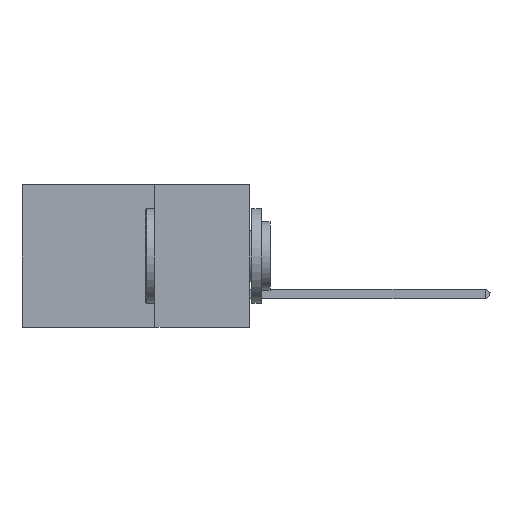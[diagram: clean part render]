
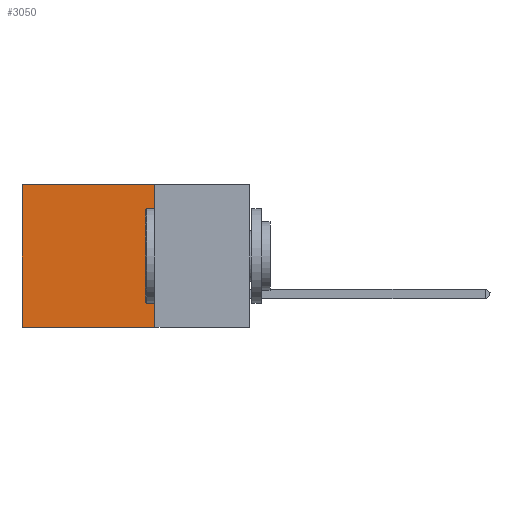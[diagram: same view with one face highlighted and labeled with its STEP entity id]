
A CAD part, left-side view. The second image highlights one B-rep face of the part: STEP entity #3050.
In plain terms, the highlighted planar face has unit normal (-1, 0, 0).
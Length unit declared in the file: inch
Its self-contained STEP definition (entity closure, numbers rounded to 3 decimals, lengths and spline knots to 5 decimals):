
#514 = DIRECTION ( 'NONE',  ( 0., 0., -1. ) ) ;
#1118 = VECTOR ( 'NONE', #9694, 39.37008 ) ;
#1240 = CARTESIAN_POINT ( 'NONE',  ( 0.2875, 0.6, -0.375 ) ) ;
#1529 = ORIENTED_EDGE ( 'NONE', *, *, #11864, .F. ) ;
#1960 = VERTEX_POINT ( 'NONE', #14443 ) ;
#3050 = ADVANCED_FACE ( 'NONE', ( #8860 ), #10366, .F. ) ;
#4208 = EDGE_LOOP ( 'NONE', ( #14770, #6728, #1529, #16789 ) ) ;
#4593 = CARTESIAN_POINT ( 'NONE',  ( 0.2875, 0.25, -0.375 ) ) ;
#5325 = EDGE_CURVE ( 'NONE', #17146, #1960, #9443, .T. ) ;
#5457 = CARTESIAN_POINT ( 'NONE',  ( 0.2875, 0.25, 0. ) ) ;
#6728 = ORIENTED_EDGE ( 'NONE', *, *, #14338, .F. ) ;
#6798 = CARTESIAN_POINT ( 'NONE',  ( 0.2875, 0.25, 0. ) ) ;
#7000 = AXIS2_PLACEMENT_3D ( 'NONE', #9120, #14892, #514 ) ;
#7699 = VERTEX_POINT ( 'NONE', #15170 ) ;
#7794 = CARTESIAN_POINT ( 'NONE',  ( 0.2875, 0.25, -0.375 ) ) ;
#7852 = VECTOR ( 'NONE', #16103, 39.37008 ) ;
#8070 = VERTEX_POINT ( 'NONE', #7794 ) ;
#8860 = FACE_OUTER_BOUND ( 'NONE', #4208, .T. ) ;
#9120 = CARTESIAN_POINT ( 'NONE',  ( 0.2875, 0.25, -0.375 ) ) ;
#9443 = LINE ( 'NONE', #6798, #1118 ) ;
#9694 = DIRECTION ( 'NONE',  ( 0., 1., 0. ) ) ;
#9783 = DIRECTION ( 'NONE',  ( 0., 0., -1. ) ) ;
#9868 = VECTOR ( 'NONE', #9783, 39.37008 ) ;
#10366 = PLANE ( 'NONE',  #7000 ) ;
#11656 = VECTOR ( 'NONE', #17622, 39.37008 ) ;
#11864 = EDGE_CURVE ( 'NONE', #17146, #8070, #16835, .T. ) ;
#12086 = LINE ( 'NONE', #1240, #9868 ) ;
#12110 = LINE ( 'NONE', #17755, #11656 ) ;
#12317 = EDGE_CURVE ( 'NONE', #1960, #7699, #12086, .T. ) ;
#14338 = EDGE_CURVE ( 'NONE', #8070, #7699, #12110, .T. ) ;
#14443 = CARTESIAN_POINT ( 'NONE',  ( 0.2875, 0.6, 0. ) ) ;
#14770 = ORIENTED_EDGE ( 'NONE', *, *, #12317, .T. ) ;
#14892 = DIRECTION ( 'NONE',  ( 1., 0., 0. ) ) ;
#15170 = CARTESIAN_POINT ( 'NONE',  ( 0.2875, 0.6, -0.375 ) ) ;
#16103 = DIRECTION ( 'NONE',  ( 0., 0., -1. ) ) ;
#16789 = ORIENTED_EDGE ( 'NONE', *, *, #5325, .T. ) ;
#16835 = LINE ( 'NONE', #4593, #7852 ) ;
#17146 = VERTEX_POINT ( 'NONE', #5457 ) ;
#17622 = DIRECTION ( 'NONE',  ( 0., 1., 0. ) ) ;
#17755 = CARTESIAN_POINT ( 'NONE',  ( 0.2875, 0.25, -0.375 ) ) ;
